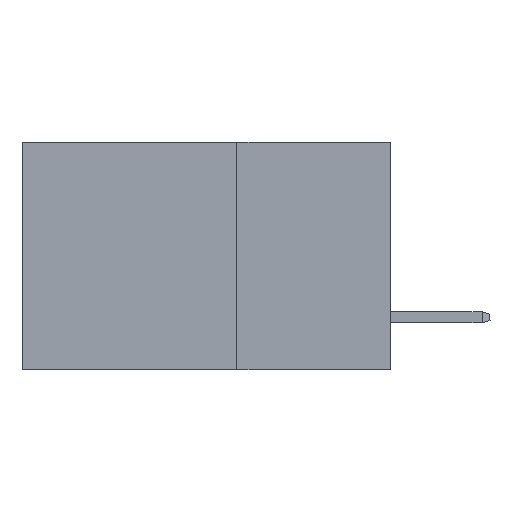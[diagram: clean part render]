
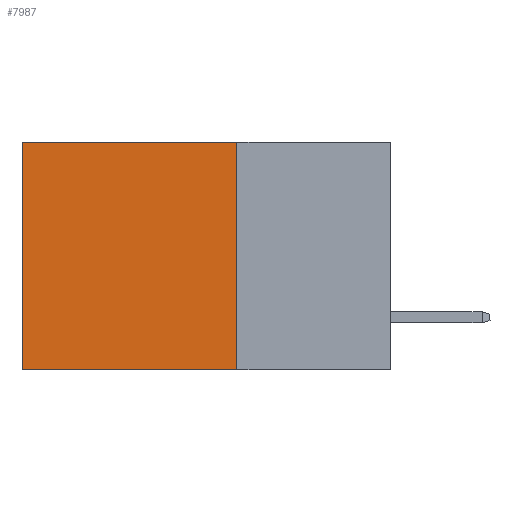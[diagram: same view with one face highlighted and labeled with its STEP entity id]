
A CAD part, left-side view. The second image highlights one B-rep face of the part: STEP entity #7987.
In plain terms, the highlighted planar face has unit normal (-1, 0, 0).
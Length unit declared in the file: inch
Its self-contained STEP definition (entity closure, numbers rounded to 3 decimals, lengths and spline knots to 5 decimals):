
#236 = CARTESIAN_POINT ( 'NONE',  ( 0.2875, 0.25, 0. ) ) ;
#432 = CARTESIAN_POINT ( 'NONE',  ( 0.2875, 0.6, 0. ) ) ;
#1375 = EDGE_CURVE ( 'NONE', #3925, #3607, #2335, .T. ) ;
#1431 = DIRECTION ( 'NONE',  ( 0., 0., -1. ) ) ;
#1553 = VECTOR ( 'NONE', #1431, 39.37008 ) ;
#2183 = CARTESIAN_POINT ( 'NONE',  ( 0.2875, 0.25, 0. ) ) ;
#2335 = LINE ( 'NONE', #2183, #4793 ) ;
#2535 = VERTEX_POINT ( 'NONE', #432 ) ;
#2662 = FACE_OUTER_BOUND ( 'NONE', #7106, .T. ) ;
#3412 = CARTESIAN_POINT ( 'NONE',  ( 0.2875, 0.25, 0. ) ) ;
#3607 = VERTEX_POINT ( 'NONE', #7109 ) ;
#3713 = ORIENTED_EDGE ( 'NONE', *, *, #1375, .F. ) ;
#3815 = ORIENTED_EDGE ( 'NONE', *, *, #8285, .F. ) ;
#3925 = VERTEX_POINT ( 'NONE', #236 ) ;
#3933 = PLANE ( 'NONE',  #9092 ) ;
#4199 = ORIENTED_EDGE ( 'NONE', *, *, #5786, .T. ) ;
#4539 = LINE ( 'NONE', #5549, #1553 ) ;
#4793 = VECTOR ( 'NONE', #7931, 39.37008 ) ;
#5549 = CARTESIAN_POINT ( 'NONE',  ( 0.2875, 0.6, 0. ) ) ;
#5786 = EDGE_CURVE ( 'NONE', #2535, #7487, #4539, .T. ) ;
#6063 = VECTOR ( 'NONE', #8460, 39.37008 ) ;
#6291 = DIRECTION ( 'NONE',  ( 0., 0., -1. ) ) ;
#6358 = CARTESIAN_POINT ( 'NONE',  ( 0.2875, 0.25, 0. ) ) ;
#6661 = CARTESIAN_POINT ( 'NONE',  ( 0.2875, 0.25, -0.37 ) ) ;
#7089 = DIRECTION ( 'NONE',  ( 1., 0., 0. ) ) ;
#7106 = EDGE_LOOP ( 'NONE', ( #4199, #3815, #3713, #9964 ) ) ;
#7109 = CARTESIAN_POINT ( 'NONE',  ( 0.2875, 0.25, -0.37 ) ) ;
#7236 = LINE ( 'NONE', #6661, #8015 ) ;
#7487 = VERTEX_POINT ( 'NONE', #8797 ) ;
#7931 = DIRECTION ( 'NONE',  ( 0., 0., -1. ) ) ;
#7987 = ADVANCED_FACE ( 'NONE', ( #2662 ), #3933, .F. ) ;
#8015 = VECTOR ( 'NONE', #9110, 39.37008 ) ;
#8285 = EDGE_CURVE ( 'NONE', #3607, #7487, #7236, .T. ) ;
#8460 = DIRECTION ( 'NONE',  ( 0., 1., 0. ) ) ;
#8797 = CARTESIAN_POINT ( 'NONE',  ( 0.2875, 0.6, -0.37 ) ) ;
#8919 = LINE ( 'NONE', #3412, #6063 ) ;
#9092 = AXIS2_PLACEMENT_3D ( 'NONE', #6358, #7089, #6291 ) ;
#9110 = DIRECTION ( 'NONE',  ( 0., 1., 0. ) ) ;
#9964 = ORIENTED_EDGE ( 'NONE', *, *, #10082, .T. ) ;
#10082 = EDGE_CURVE ( 'NONE', #3925, #2535, #8919, .T. ) ;
